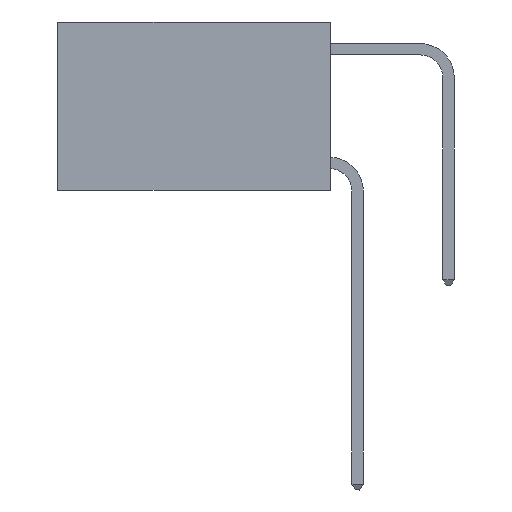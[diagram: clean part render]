
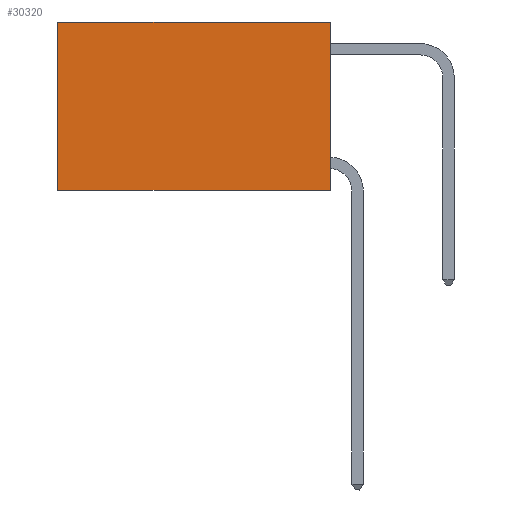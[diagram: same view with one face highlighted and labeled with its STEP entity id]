
A CAD part, left-side view. The second image highlights one B-rep face of the part: STEP entity #30320.
In plain terms, the highlighted planar face has unit normal (-1, 0, 0).
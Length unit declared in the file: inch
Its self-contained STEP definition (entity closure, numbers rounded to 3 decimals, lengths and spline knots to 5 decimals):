
#332 = VERTEX_POINT ( 'NONE', #13028 ) ;
#1085 = DIRECTION ( 'NONE',  ( 0., 0., -1. ) ) ;
#2125 = AXIS2_PLACEMENT_3D ( 'NONE', #5973, #8317, #10670 ) ;
#3113 = FACE_OUTER_BOUND ( 'NONE', #13935, .T. ) ;
#3436 = CARTESIAN_POINT ( 'NONE',  ( 0.2625, 0., 0. ) ) ;
#3963 = ORIENTED_EDGE ( 'NONE', *, *, #19057, .T. ) ;
#5454 = LINE ( 'NONE', #25564, #28721 ) ;
#5669 = CARTESIAN_POINT ( 'NONE',  ( 0.2625, 0., -0.37 ) ) ;
#5871 = DIRECTION ( 'NONE',  ( 0., 1., 0. ) ) ;
#5973 = CARTESIAN_POINT ( 'NONE',  ( 0.2625, 0., 0. ) ) ;
#6272 = CARTESIAN_POINT ( 'NONE',  ( 0.2625, 0., -0.37 ) ) ;
#6667 = LINE ( 'NONE', #12725, #18804 ) ;
#8317 = DIRECTION ( 'NONE',  ( 1., 0., 0. ) ) ;
#9258 = ORIENTED_EDGE ( 'NONE', *, *, #19132, .F. ) ;
#10670 = DIRECTION ( 'NONE',  ( 0., 0., -1. ) ) ;
#11007 = VERTEX_POINT ( 'NONE', #6272 ) ;
#11054 = LINE ( 'NONE', #5669, #11776 ) ;
#11262 = EDGE_CURVE ( 'NONE', #19149, #332, #23861, .T. ) ;
#11776 = VECTOR ( 'NONE', #5871, 39.37008 ) ;
#12019 = VECTOR ( 'NONE', #24393, 39.37008 ) ;
#12725 = CARTESIAN_POINT ( 'NONE',  ( 0.2625, 0.6, 0. ) ) ;
#13028 = CARTESIAN_POINT ( 'NONE',  ( 0.2625, 0.6, 0. ) ) ;
#13935 = EDGE_LOOP ( 'NONE', ( #3963, #9258, #24568, #22309 ) ) ;
#15305 = PLANE ( 'NONE',  #2125 ) ;
#18629 = DIRECTION ( 'NONE',  ( 0., 0., -1. ) ) ;
#18804 = VECTOR ( 'NONE', #1085, 39.37008 ) ;
#19057 = EDGE_CURVE ( 'NONE', #332, #26028, #6667, .T. ) ;
#19132 = EDGE_CURVE ( 'NONE', #11007, #26028, #11054, .T. ) ;
#19149 = VERTEX_POINT ( 'NONE', #3436 ) ;
#20345 = CARTESIAN_POINT ( 'NONE',  ( 0.2625, 0.6, -0.37 ) ) ;
#21730 = CARTESIAN_POINT ( 'NONE',  ( 0.2625, 0., 0. ) ) ;
#22309 = ORIENTED_EDGE ( 'NONE', *, *, #11262, .T. ) ;
#23861 = LINE ( 'NONE', #21730, #12019 ) ;
#24393 = DIRECTION ( 'NONE',  ( 0., 1., 0. ) ) ;
#24568 = ORIENTED_EDGE ( 'NONE', *, *, #26179, .F. ) ;
#25564 = CARTESIAN_POINT ( 'NONE',  ( 0.2625, 0., 0. ) ) ;
#26028 = VERTEX_POINT ( 'NONE', #20345 ) ;
#26179 = EDGE_CURVE ( 'NONE', #19149, #11007, #5454, .T. ) ;
#28721 = VECTOR ( 'NONE', #18629, 39.37008 ) ;
#30320 = ADVANCED_FACE ( 'NONE', ( #3113 ), #15305, .F. ) ;
